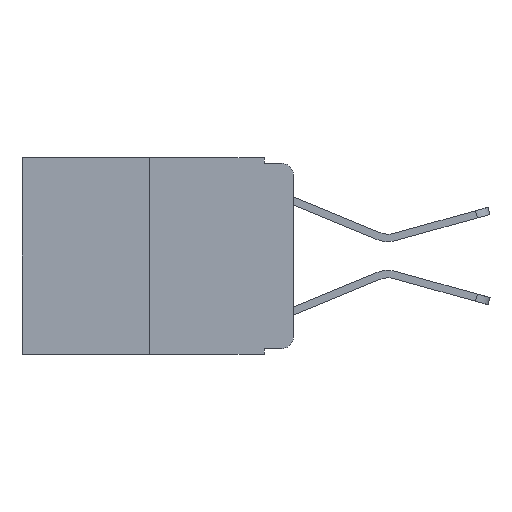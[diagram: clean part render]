
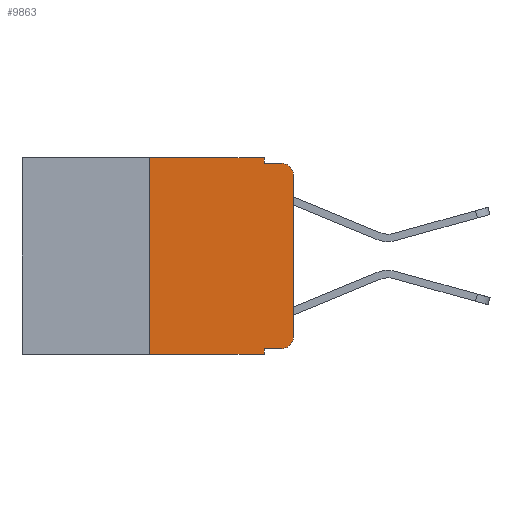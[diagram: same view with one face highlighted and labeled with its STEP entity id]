
A CAD part, left-side view. The second image highlights one B-rep face of the part: STEP entity #9863.
In plain terms, the highlighted planar face has unit normal (-1, 0, 0).
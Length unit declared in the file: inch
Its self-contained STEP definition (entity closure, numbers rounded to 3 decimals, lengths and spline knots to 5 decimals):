
#21 = EDGE_LOOP ( 'NONE', ( #4349, #2112, #1193, #10882, #9232, #10075, #1450, #1766, #8365, #10424 ) ) ;
#461 = CARTESIAN_POINT ( 'NONE',  ( 0., 0.051, -0.01 ) ) ;
#771 = PLANE ( 'NONE',  #9424 ) ;
#973 = LINE ( 'NONE', #4875, #8132 ) ;
#1042 = EDGE_CURVE ( 'NONE', #7828, #6786, #10523, .T. ) ;
#1193 = ORIENTED_EDGE ( 'NONE', *, *, #8318, .F. ) ;
#1336 = CARTESIAN_POINT ( 'NONE',  ( 0., 0.051, -0.343 ) ) ;
#1450 = ORIENTED_EDGE ( 'NONE', *, *, #1042, .T. ) ;
#1515 = EDGE_CURVE ( 'NONE', #11468, #7976, #9470, .T. ) ;
#1572 = LINE ( 'NONE', #3690, #10972 ) ;
#1698 = CARTESIAN_POINT ( 'NONE',  ( 0., 0.051, -0.333 ) ) ;
#1766 = ORIENTED_EDGE ( 'NONE', *, *, #1909, .F. ) ;
#1771 = VERTEX_POINT ( 'NONE', #4209 ) ;
#1909 = EDGE_CURVE ( 'NONE', #8661, #6786, #4901, .T. ) ;
#2060 = CARTESIAN_POINT ( 'NONE',  ( 0., 0., -0.313 ) ) ;
#2112 = ORIENTED_EDGE ( 'NONE', *, *, #5325, .T. ) ;
#2142 = CARTESIAN_POINT ( 'NONE',  ( 0., 0.25, 0. ) ) ;
#2513 = DIRECTION ( 'NONE',  ( 0., 0., 1. ) ) ;
#2998 = DIRECTION ( 'NONE',  ( 0., 0., -1. ) ) ;
#3179 = VERTEX_POINT ( 'NONE', #6316 ) ;
#3690 = CARTESIAN_POINT ( 'NONE',  ( 0., 0.25, 0. ) ) ;
#4203 = VECTOR ( 'NONE', #4339, 39.37008 ) ;
#4209 = CARTESIAN_POINT ( 'NONE',  ( 0., 0., -0.03 ) ) ;
#4261 = DIRECTION ( 'NONE',  ( 0., -1., 0. ) ) ;
#4339 = DIRECTION ( 'NONE',  ( 0., -1., 0. ) ) ;
#4349 = ORIENTED_EDGE ( 'NONE', *, *, #7814, .T. ) ;
#4381 = DIRECTION ( 'NONE',  ( -1., 0., 0. ) ) ;
#4403 = EDGE_CURVE ( 'NONE', #11319, #3179, #973, .T. ) ;
#4737 = FACE_OUTER_BOUND ( 'NONE', #21, .T. ) ;
#4848 = CARTESIAN_POINT ( 'NONE',  ( 0., 0.02, -0.313 ) ) ;
#4875 = CARTESIAN_POINT ( 'NONE',  ( 0., 0.473, 0. ) ) ;
#4901 = LINE ( 'NONE', #9011, #8054 ) ;
#4930 = LINE ( 'NONE', #6185, #8214 ) ;
#5153 = EDGE_CURVE ( 'NONE', #3179, #10831, #6676, .T. ) ;
#5221 = VECTOR ( 'NONE', #4261, 39.37008 ) ;
#5325 = EDGE_CURVE ( 'NONE', #1771, #6064, #10795, .T. ) ;
#5753 = CARTESIAN_POINT ( 'NONE',  ( 0., 0.473, -0.343 ) ) ;
#5974 = AXIS2_PLACEMENT_3D ( 'NONE', #9950, #4381, #10787 ) ;
#6064 = VERTEX_POINT ( 'NONE', #10744 ) ;
#6185 = CARTESIAN_POINT ( 'NONE',  ( 0., 0., 0. ) ) ;
#6316 = CARTESIAN_POINT ( 'NONE',  ( 0., 0.051, 0. ) ) ;
#6531 = DIRECTION ( 'NONE',  ( -1., 0., 0. ) ) ;
#6676 = LINE ( 'NONE', #8646, #8515 ) ;
#6786 = VERTEX_POINT ( 'NONE', #1336 ) ;
#7157 = DIRECTION ( 'NONE',  ( 1., 0., 0. ) ) ;
#7196 = LINE ( 'NONE', #10352, #4203 ) ;
#7208 = LINE ( 'NONE', #9762, #5221 ) ;
#7275 = EDGE_CURVE ( 'NONE', #8661, #11468, #7208, .T. ) ;
#7814 = EDGE_CURVE ( 'NONE', #7976, #1771, #4930, .T. ) ;
#7828 = VERTEX_POINT ( 'NONE', #9812 ) ;
#7976 = VERTEX_POINT ( 'NONE', #2060 ) ;
#8054 = VECTOR ( 'NONE', #10851, 39.37008 ) ;
#8098 = DIRECTION ( 'NONE',  ( 0., 0., -1. ) ) ;
#8118 = VECTOR ( 'NONE', #9524, 39.37008 ) ;
#8132 = VECTOR ( 'NONE', #10488, 39.37008 ) ;
#8214 = VECTOR ( 'NONE', #2513, 39.37008 ) ;
#8318 = EDGE_CURVE ( 'NONE', #10831, #6064, #7196, .T. ) ;
#8365 = ORIENTED_EDGE ( 'NONE', *, *, #7275, .T. ) ;
#8515 = VECTOR ( 'NONE', #8601, 39.37008 ) ;
#8601 = DIRECTION ( 'NONE',  ( 0., 0., -1. ) ) ;
#8646 = CARTESIAN_POINT ( 'NONE',  ( 0., 0.051, 0. ) ) ;
#8661 = VERTEX_POINT ( 'NONE', #1698 ) ;
#9011 = CARTESIAN_POINT ( 'NONE',  ( 0., 0.051, 0. ) ) ;
#9061 = AXIS2_PLACEMENT_3D ( 'NONE', #4848, #6531, #2998 ) ;
#9232 = ORIENTED_EDGE ( 'NONE', *, *, #4403, .F. ) ;
#9424 = AXIS2_PLACEMENT_3D ( 'NONE', #10857, #7157, #8098 ) ;
#9470 = CIRCLE ( 'NONE', #9061, 0.02 ) ;
#9524 = DIRECTION ( 'NONE',  ( 0., -1., 0. ) ) ;
#9715 = CARTESIAN_POINT ( 'NONE',  ( 0., 0.02, -0.333 ) ) ;
#9762 = CARTESIAN_POINT ( 'NONE',  ( 0., 0.051, -0.333 ) ) ;
#9812 = CARTESIAN_POINT ( 'NONE',  ( 0., 0.25, -0.343 ) ) ;
#9863 = ADVANCED_FACE ( 'NONE', ( #4737 ), #771, .F. ) ;
#9950 = CARTESIAN_POINT ( 'NONE',  ( 0., 0.02, -0.03 ) ) ;
#10075 = ORIENTED_EDGE ( 'NONE', *, *, #11099, .F. ) ;
#10352 = CARTESIAN_POINT ( 'NONE',  ( 0., 0.051, -0.01 ) ) ;
#10424 = ORIENTED_EDGE ( 'NONE', *, *, #1515, .T. ) ;
#10488 = DIRECTION ( 'NONE',  ( 0., -1., 0. ) ) ;
#10523 = LINE ( 'NONE', #5753, #8118 ) ;
#10744 = CARTESIAN_POINT ( 'NONE',  ( 0., 0.02, -0.01 ) ) ;
#10787 = DIRECTION ( 'NONE',  ( 0., 0., -1. ) ) ;
#10795 = CIRCLE ( 'NONE', #5974, 0.02 ) ;
#10831 = VERTEX_POINT ( 'NONE', #461 ) ;
#10851 = DIRECTION ( 'NONE',  ( 0., 0., -1. ) ) ;
#10857 = CARTESIAN_POINT ( 'NONE',  ( 0., 0.473, 0. ) ) ;
#10882 = ORIENTED_EDGE ( 'NONE', *, *, #5153, .F. ) ;
#10972 = VECTOR ( 'NONE', #10986, 39.37008 ) ;
#10986 = DIRECTION ( 'NONE',  ( 0., 0., 1. ) ) ;
#11099 = EDGE_CURVE ( 'NONE', #7828, #11319, #1572, .T. ) ;
#11319 = VERTEX_POINT ( 'NONE', #2142 ) ;
#11468 = VERTEX_POINT ( 'NONE', #9715 ) ;
